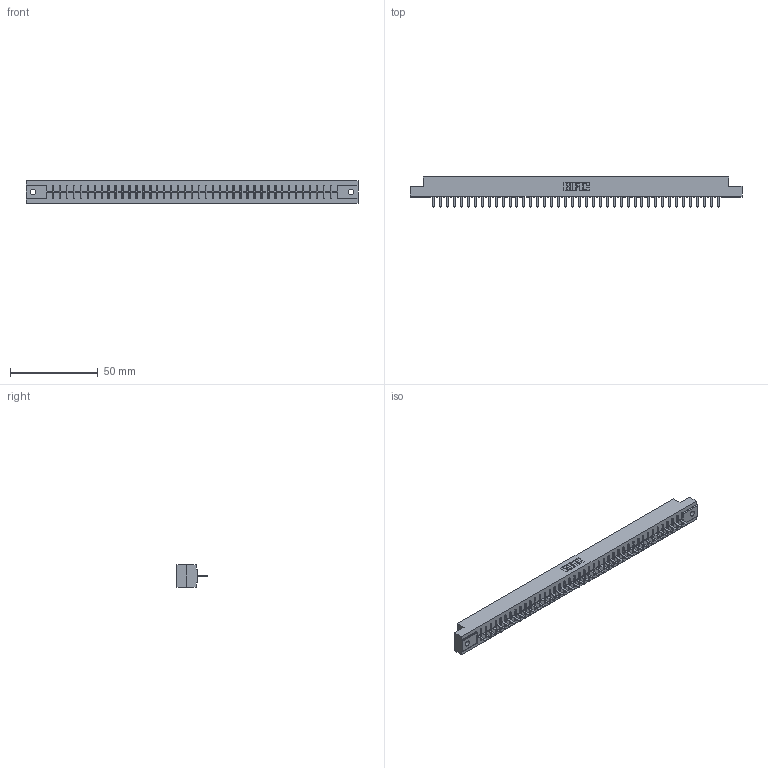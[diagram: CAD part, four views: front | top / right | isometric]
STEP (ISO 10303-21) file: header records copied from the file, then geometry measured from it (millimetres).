
FILE_DESCRIPTION (( 'STEP AP203' ), '1' );
FILE_NAME ('316-042-420-102.STEP', '2020-09-23T07:31:14', ( '' ), ( '' ), 'SwSTEP 2.0', 'SolidWorks 2020', '' );
FILE_SCHEMA (( 'CONFIG_CONTROL_DESIGN' ));
Length unit declared in the file: inch
Products named in the file (3): 306 Part_.128 Dia; 316-042-420-102; 306-290-001_120
Assembly tree (43 placements, depth 2):
  316-042-420-102
    306 Part_.128 Dia
    306-290-001_120  x42
Bounding box: 189.43 x 17.12 x 12.7 mm (x, y, z)
Volume: 20926.9 mm3; surface area: 21208.2 mm2
Topology: 43 solids, 43 shells, 3056 faces, 8590 edges, 5500 vertices
Faces by surface type: plane 2042, cylinder 846, sphere 168
Entity records: 39125 total; most frequent: CARTESIAN_POINT 6569, ORIENTED_EDGE 6512, DIRECTION 6478, EDGE_CURVE 3256, VECTOR 2548, LINE 2548, VERTEX_POINT 2056, AXIS2_PLACEMENT_3D 1965
